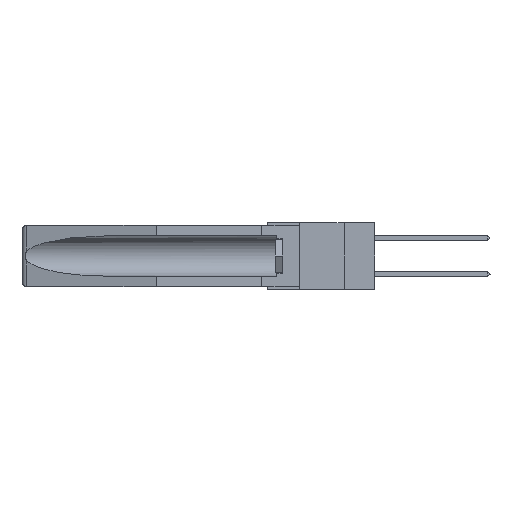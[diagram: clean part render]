
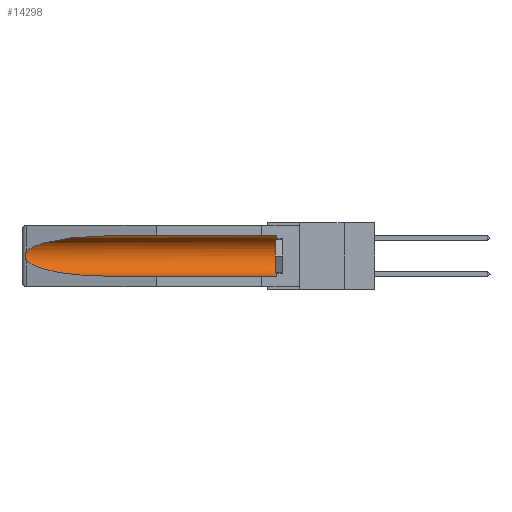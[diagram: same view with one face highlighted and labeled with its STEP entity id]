
A CAD part, left-side view. The second image highlights one B-rep face of the part: STEP entity #14298.
In plain terms, the highlighted cylindrical face has radius 2.857 mm (diameter 5.715 mm), a partial arc.
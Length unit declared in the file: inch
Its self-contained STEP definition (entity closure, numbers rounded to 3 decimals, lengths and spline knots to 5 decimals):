
#250 = ORIENTED_EDGE ( 'NONE', *, *, #15411, .T. ) ;
#333 = VERTEX_POINT ( 'NONE', #19420 ) ;
#478 = CARTESIAN_POINT ( 'NONE',  ( 0.155, 0.126, -0.059 ) ) ;
#760 = EDGE_CURVE ( 'NONE', #14365, #6909, #14109, .T. ) ;
#974 = ORIENTED_EDGE ( 'NONE', *, *, #1298, .T. ) ;
#1192 = VERTEX_POINT ( 'NONE', #6560 ) ;
#1298 = EDGE_CURVE ( 'NONE', #14365, #3651, #4731, .T. ) ;
#1502 = VERTEX_POINT ( 'NONE', #18621 ) ;
#1597 = CARTESIAN_POINT ( 'NONE',  ( 0.26537, 1.52718, -0.19328 ) ) ;
#2438 = CARTESIAN_POINT ( 'NONE',  ( 0.2673, 1.5327, -0.16383 ) ) ;
#3470 = CARTESIAN_POINT ( 'NONE',  ( 0.155, 1.07973, -0.284 ) ) ;
#3518 = DIRECTION ( 'NONE',  ( 0., 1., 0. ) ) ;
#3651 = VERTEX_POINT ( 'NONE', #478 ) ;
#3739 = DIRECTION ( 'NONE',  ( 0., 0., 1. ) ) ;
#3906 = CARTESIAN_POINT ( 'NONE',  ( 0.26537, 1.52718, -0.14972 ) ) ;
#3983 = CARTESIAN_POINT ( 'NONE',  ( 0.26597, 1.52961, -0.15275 ) ) ;
#4052 = CARTESIAN_POINT ( 'NONE',  ( 0.2675, 1.53308, -0.17534 ) ) ;
#4192 = EDGE_CURVE ( 'NONE', #333, #1192, #18014, .T. ) ;
#4384 = CARTESIAN_POINT ( 'NONE',  ( 0.21114, 1.30732, -0.059 ) ) ;
#4731 = CIRCLE ( 'NONE', #5276, 0.1125 ) ;
#5276 = AXIS2_PLACEMENT_3D ( 'NONE', #20909, #15891, #5901 ) ;
#5711 = CARTESIAN_POINT ( 'NONE',  ( 0.26655, 1.53094, -0.18657 ) ) ;
#5901 = DIRECTION ( 'NONE',  ( 0., 0., 1. ) ) ;
#5957 = EDGE_CURVE ( 'NONE', #1192, #6909, #10221, .T. ) ;
#6560 = CARTESIAN_POINT ( 'NONE',  ( 0.26537, 1.52718, -0.19328 ) ) ;
#6909 = VERTEX_POINT ( 'NONE', #11904 ) ;
#7231 = CARTESIAN_POINT ( 'NONE',  ( 0.2673, 1.53269, -0.17917 ) ) ;
#8221 = CARTESIAN_POINT ( 'NONE',  ( 0.25451, 1.48313, -0.09465 ) ) ;
#8732 = ORIENTED_EDGE ( 'NONE', *, *, #5957, .T. ) ;
#9163 = CARTESIAN_POINT ( 'NONE',  ( 0.26597, 1.5296, -0.19026 ) ) ;
#9483 = ORIENTED_EDGE ( 'NONE', *, *, #15090, .T. ) ;
#9952 = LINE ( 'NONE', #10311, #16245 ) ;
#10053 = CARTESIAN_POINT ( 'NONE',  ( 0.25451, 1.48313, -0.24835 ) ) ;
#10221 =( BOUNDED_CURVE ( )  B_SPLINE_CURVE ( 3, ( #1597, #10053, #11709, #3470 ),
 .UNSPECIFIED., .F., .F. ) 
 B_SPLINE_CURVE_WITH_KNOTS ( ( 4, 4 ),
 ( 0.1948, 1.5708 ),
 .UNSPECIFIED. ) 
 CURVE ( )  GEOMETRIC_REPRESENTATION_ITEM ( )  RATIONAL_B_SPLINE_CURVE ( ( 1., 0.848, 0.848, 1. ) ) 
 REPRESENTATION_ITEM ( '' )  );
#10311 = CARTESIAN_POINT ( 'NONE',  ( 0.155, -0.30754, -0.059 ) ) ;
#11011 =( BOUNDED_CURVE ( )  B_SPLINE_CURVE ( 3, ( #14184, #4384, #8221, #13518 ),
 .UNSPECIFIED., .F., .F. ) 
 B_SPLINE_CURVE_WITH_KNOTS ( ( 4, 4 ),
 ( 4.71239, 6.08839 ),
 .UNSPECIFIED. ) 
 CURVE ( )  GEOMETRIC_REPRESENTATION_ITEM ( )  RATIONAL_B_SPLINE_CURVE ( ( 1., 0.848, 0.848, 1. ) ) 
 REPRESENTATION_ITEM ( '' )  );
#11464 = VECTOR ( 'NONE', #19555, 39.37008 ) ;
#11709 = CARTESIAN_POINT ( 'NONE',  ( 0.21114, 1.30732, -0.284 ) ) ;
#11904 = CARTESIAN_POINT ( 'NONE',  ( 0.155, 1.07973, -0.284 ) ) ;
#11961 = EDGE_LOOP ( 'NONE', ( #250, #17084, #8732, #18868, #974, #9483 ) ) ;
#12847 = FACE_OUTER_BOUND ( 'NONE', #11961, .T. ) ;
#13518 = CARTESIAN_POINT ( 'NONE',  ( 0.26537, 1.52718, -0.14972 ) ) ;
#14064 = CARTESIAN_POINT ( 'NONE',  ( 0.2675, 1.53308, -0.16763 ) ) ;
#14109 = LINE ( 'NONE', #14497, #11464 ) ;
#14184 = CARTESIAN_POINT ( 'NONE',  ( 0.155, 1.07973, -0.059 ) ) ;
#14298 = ADVANCED_FACE ( 'NONE', ( #12847 ), #20205, .F. ) ;
#14365 = VERTEX_POINT ( 'NONE', #17223 ) ;
#14407 = AXIS2_PLACEMENT_3D ( 'NONE', #17080, #18663, #3739 ) ;
#14497 = CARTESIAN_POINT ( 'NONE',  ( 0.155, -0.30754, -0.284 ) ) ;
#15090 = EDGE_CURVE ( 'NONE', #3651, #1502, #9952, .T. ) ;
#15411 = EDGE_CURVE ( 'NONE', #1502, #333, #11011, .T. ) ;
#15891 = DIRECTION ( 'NONE',  ( 0., -1., 0. ) ) ;
#16245 = VECTOR ( 'NONE', #3518, 39.37008 ) ;
#17080 = CARTESIAN_POINT ( 'NONE',  ( 0.155, -0.30754, -0.1715 ) ) ;
#17084 = ORIENTED_EDGE ( 'NONE', *, *, #4192, .T. ) ;
#17223 = CARTESIAN_POINT ( 'NONE',  ( 0.155, 0.126, -0.284 ) ) ;
#17241 = CARTESIAN_POINT ( 'NONE',  ( 0.26654, 1.53092, -0.15636 ) ) ;
#18014 = B_SPLINE_CURVE_WITH_KNOTS ( 'NONE', 3,
 ( #3906, #3983, #17241, #2438, #14064, #4052, #7231, #5711, #9163, #20874 ),
 .UNSPECIFIED., .F., .F.,
 ( 4, 2, 2, 2, 4 ),
 ( 0., 0.00029, 0.00058, 0.00087, 0.00117 ),
 .UNSPECIFIED. ) ;
#18621 = CARTESIAN_POINT ( 'NONE',  ( 0.155, 1.07973, -0.059 ) ) ;
#18663 = DIRECTION ( 'NONE',  ( 0., 1., 0. ) ) ;
#18868 = ORIENTED_EDGE ( 'NONE', *, *, #760, .F. ) ;
#19420 = CARTESIAN_POINT ( 'NONE',  ( 0.26537, 1.52718, -0.14972 ) ) ;
#19555 = DIRECTION ( 'NONE',  ( 0., 1., 0. ) ) ;
#20205 = CYLINDRICAL_SURFACE ( 'NONE', #14407, 0.1125 ) ;
#20874 = CARTESIAN_POINT ( 'NONE',  ( 0.26537, 1.52718, -0.19328 ) ) ;
#20909 = CARTESIAN_POINT ( 'NONE',  ( 0.155, 0.126, -0.1715 ) ) ;
